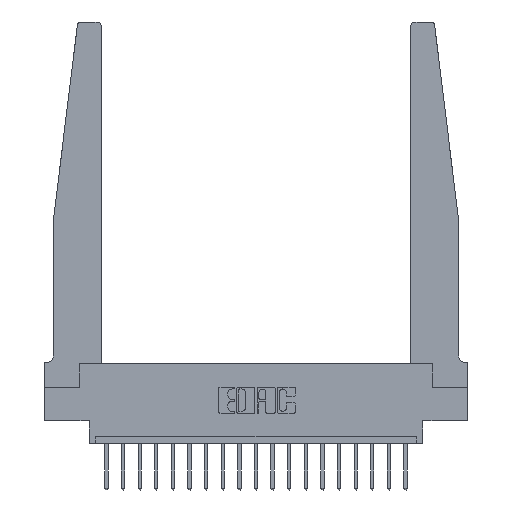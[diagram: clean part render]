
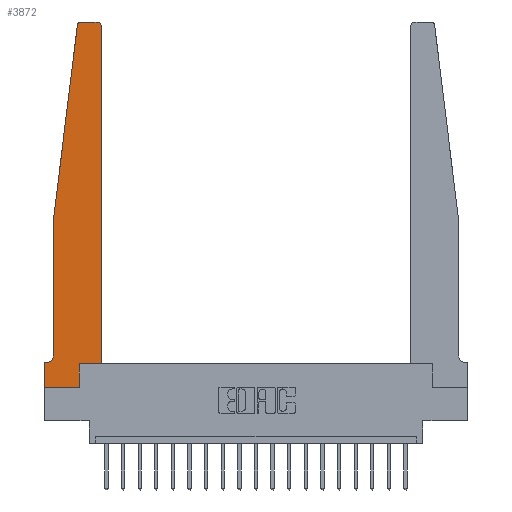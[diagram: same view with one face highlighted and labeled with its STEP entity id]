
A CAD part, top view. The second image highlights one B-rep face of the part: STEP entity #3872.
In plain terms, the highlighted planar face has unit normal (0, 0, 1).
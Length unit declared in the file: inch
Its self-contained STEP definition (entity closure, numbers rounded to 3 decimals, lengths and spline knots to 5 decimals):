
#83 = CARTESIAN_POINT ( 'NONE',  ( 0.24675, 2.72367, 0.37 ) ) ;
#197 = CARTESIAN_POINT ( 'NONE',  ( 0., 0.1875, 0.37 ) ) ;
#530 = DIRECTION ( 'NONE',  ( 0., 0., 1. ) ) ;
#598 = EDGE_CURVE ( 'NONE', #7718, #3183, #7054, .T. ) ;
#789 = CARTESIAN_POINT ( 'NONE',  ( 0.065, 0.2375, 0.37 ) ) ;
#822 = AXIS2_PLACEMENT_3D ( 'NONE', #4250, #17074, #19979 ) ;
#1014 = EDGE_CURVE ( 'NONE', #5864, #8013, #8455, .T. ) ;
#1153 = ORIENTED_EDGE ( 'NONE', *, *, #1014, .T. ) ;
#1346 = ORIENTED_EDGE ( 'NONE', *, *, #16057, .T. ) ;
#1486 = ORIENTED_EDGE ( 'NONE', *, *, #4375, .T. ) ;
#1783 = CARTESIAN_POINT ( 'NONE',  ( 0.2605, 0.18, 0.37 ) ) ;
#2416 = DIRECTION ( 'NONE',  ( 1., 0., 0. ) ) ;
#2803 = FACE_OUTER_BOUND ( 'NONE', #7876, .T. ) ;
#3183 = VERTEX_POINT ( 'NONE', #17340 ) ;
#3249 = AXIS2_PLACEMENT_3D ( 'NONE', #11610, #5317, #2416 ) ;
#3282 = ORIENTED_EDGE ( 'NONE', *, *, #7738, .T. ) ;
#3742 = DIRECTION ( 'NONE',  ( 0., -1., 0. ) ) ;
#3872 = ADVANCED_FACE ( 'NONE', ( #2803 ), #4653, .T. ) ;
#3971 = DIRECTION ( 'NONE',  ( 1., 0., 0. ) ) ;
#3983 = LINE ( 'NONE', #15087, #12665 ) ;
#4030 = CARTESIAN_POINT ( 'NONE',  ( 0.395, 2.72, 0.37 ) ) ;
#4070 = VECTOR ( 'NONE', #3742, 39.37008 ) ;
#4130 = CARTESIAN_POINT ( 'NONE',  ( 0.015, 0.2375, 0.37 ) ) ;
#4250 = CARTESIAN_POINT ( 'NONE',  ( 0., 0.1875, 0.37 ) ) ;
#4313 = CARTESIAN_POINT ( 'NONE',  ( 0.25, 2.75, 0.37 ) ) ;
#4375 = EDGE_CURVE ( 'NONE', #7959, #6542, #18395, .T. ) ;
#4637 = DIRECTION ( 'NONE',  ( 0., -1., 0. ) ) ;
#4646 = EDGE_CURVE ( 'NONE', #3183, #7959, #5672, .T. ) ;
#4653 = PLANE ( 'NONE',  #822 ) ;
#4674 = VERTEX_POINT ( 'NONE', #17902 ) ;
#4858 = ORIENTED_EDGE ( 'NONE', *, *, #598, .T. ) ;
#5317 = DIRECTION ( 'NONE',  ( 0., 0., 1. ) ) ;
#5398 = VERTEX_POINT ( 'NONE', #14469 ) ;
#5672 = LINE ( 'NONE', #10343, #4070 ) ;
#5864 = VERTEX_POINT ( 'NONE', #11281 ) ;
#6134 = VECTOR ( 'NONE', #15018, 39.37008 ) ;
#6542 = VERTEX_POINT ( 'NONE', #8175 ) ;
#6562 = LINE ( 'NONE', #9800, #14164 ) ;
#6569 = DIRECTION ( 'NONE',  ( 1., 0., 0. ) ) ;
#6741 = LINE ( 'NONE', #1783, #17821 ) ;
#6771 = CIRCLE ( 'NONE', #15204, 0.03 ) ;
#7054 = LINE ( 'NONE', #13247, #18349 ) ;
#7476 = ORIENTED_EDGE ( 'NONE', *, *, #17138, .T. ) ;
#7718 = VERTEX_POINT ( 'NONE', #83 ) ;
#7738 = EDGE_CURVE ( 'NONE', #6542, #17916, #6562, .T. ) ;
#7876 = EDGE_LOOP ( 'NONE', ( #13521, #9634, #4858, #12820, #1486, #3282, #1346, #1153, #8555, #7476, #11685, #10006 ) ) ;
#7959 = VERTEX_POINT ( 'NONE', #789 ) ;
#8013 = VERTEX_POINT ( 'NONE', #10501 ) ;
#8084 = LINE ( 'NONE', #12660, #16649 ) ;
#8142 = DIRECTION ( 'NONE',  ( 0., 1., 0. ) ) ;
#8175 = CARTESIAN_POINT ( 'NONE',  ( 0.015, 0.1875, 0.37 ) ) ;
#8238 = EDGE_CURVE ( 'NONE', #9080, #7718, #13040, .T. ) ;
#8455 = LINE ( 'NONE', #14878, #19038 ) ;
#8555 = ORIENTED_EDGE ( 'NONE', *, *, #10444, .T. ) ;
#8951 = DIRECTION ( 'NONE',  ( -0.122, -0.992, 0. ) ) ;
#9015 = DIRECTION ( 'NONE',  ( -1., 0., 0. ) ) ;
#9080 = VERTEX_POINT ( 'NONE', #17097 ) ;
#9395 = DIRECTION ( 'NONE',  ( -1., 0., 0. ) ) ;
#9634 = ORIENTED_EDGE ( 'NONE', *, *, #8238, .T. ) ;
#9800 = CARTESIAN_POINT ( 'NONE',  ( 0.065, 0.1875, 0.37 ) ) ;
#9863 = EDGE_CURVE ( 'NONE', #4674, #14159, #6771, .T. ) ;
#10006 = ORIENTED_EDGE ( 'NONE', *, *, #9863, .T. ) ;
#10343 = CARTESIAN_POINT ( 'NONE',  ( 0.065, 1.25, 0.37 ) ) ;
#10444 = EDGE_CURVE ( 'NONE', #8013, #19569, #6741, .T. ) ;
#10501 = CARTESIAN_POINT ( 'NONE',  ( 0.2605, 0., 0.37 ) ) ;
#11281 = CARTESIAN_POINT ( 'NONE',  ( 0., 0., 0.37 ) ) ;
#11523 = EDGE_CURVE ( 'NONE', #14159, #9080, #12334, .T. ) ;
#11610 = CARTESIAN_POINT ( 'NONE',  ( 0.27653, 2.72, 0.37 ) ) ;
#11685 = ORIENTED_EDGE ( 'NONE', *, *, #12593, .T. ) ;
#12334 = LINE ( 'NONE', #4313, #6134 ) ;
#12440 = CARTESIAN_POINT ( 'NONE',  ( 0.2605, 0.18, 0.37 ) ) ;
#12593 = EDGE_CURVE ( 'NONE', #5398, #4674, #3983, .T. ) ;
#12660 = CARTESIAN_POINT ( 'NONE',  ( 0.425, 0.18, 0.37 ) ) ;
#12665 = VECTOR ( 'NONE', #13558, 39.37008 ) ;
#12820 = ORIENTED_EDGE ( 'NONE', *, *, #4646, .T. ) ;
#13040 = CIRCLE ( 'NONE', #3249, 0.03 ) ;
#13247 = CARTESIAN_POINT ( 'NONE',  ( 0.065, 1.25, 0.37 ) ) ;
#13521 = ORIENTED_EDGE ( 'NONE', *, *, #11523, .T. ) ;
#13558 = DIRECTION ( 'NONE',  ( 0., 1., 0. ) ) ;
#14159 = VERTEX_POINT ( 'NONE', #17104 ) ;
#14164 = VECTOR ( 'NONE', #9395, 39.37008 ) ;
#14469 = CARTESIAN_POINT ( 'NONE',  ( 0.425, 0.18, 0.37 ) ) ;
#14878 = CARTESIAN_POINT ( 'NONE',  ( 0., 0., 0.37 ) ) ;
#15018 = DIRECTION ( 'NONE',  ( -1., 0., 0. ) ) ;
#15087 = CARTESIAN_POINT ( 'NONE',  ( 0.425, 0.18, 0.37 ) ) ;
#15204 = AXIS2_PLACEMENT_3D ( 'NONE', #4030, #530, #19351 ) ;
#15329 = CARTESIAN_POINT ( 'NONE',  ( 0., 0., 0.37 ) ) ;
#16057 = EDGE_CURVE ( 'NONE', #17916, #5864, #20065, .T. ) ;
#16649 = VECTOR ( 'NONE', #6569, 39.37008 ) ;
#17074 = DIRECTION ( 'NONE',  ( 0., 0., 1. ) ) ;
#17097 = CARTESIAN_POINT ( 'NONE',  ( 0.27653, 2.75, 0.37 ) ) ;
#17104 = CARTESIAN_POINT ( 'NONE',  ( 0.395, 2.75, 0.37 ) ) ;
#17138 = EDGE_CURVE ( 'NONE', #19569, #5398, #8084, .T. ) ;
#17340 = CARTESIAN_POINT ( 'NONE',  ( 0.065, 1.25, 0.37 ) ) ;
#17726 = AXIS2_PLACEMENT_3D ( 'NONE', #4130, #20153, #9015 ) ;
#17821 = VECTOR ( 'NONE', #8142, 39.37008 ) ;
#17902 = CARTESIAN_POINT ( 'NONE',  ( 0.425, 2.72, 0.37 ) ) ;
#17916 = VERTEX_POINT ( 'NONE', #197 ) ;
#17920 = VECTOR ( 'NONE', #4637, 39.37008 ) ;
#18349 = VECTOR ( 'NONE', #8951, 39.37008 ) ;
#18395 = CIRCLE ( 'NONE', #17726, 0.05 ) ;
#19038 = VECTOR ( 'NONE', #3971, 39.37008 ) ;
#19351 = DIRECTION ( 'NONE',  ( 1., 0., 0. ) ) ;
#19569 = VERTEX_POINT ( 'NONE', #12440 ) ;
#19979 = DIRECTION ( 'NONE',  ( 1., 0., 0. ) ) ;
#20065 = LINE ( 'NONE', #15329, #17920 ) ;
#20153 = DIRECTION ( 'NONE',  ( 0., 0., -1. ) ) ;
